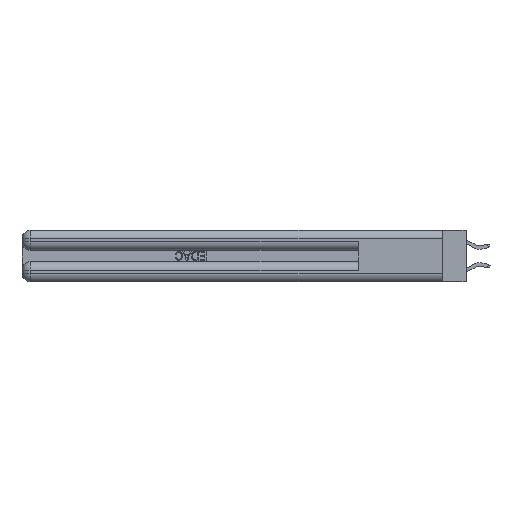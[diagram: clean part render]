
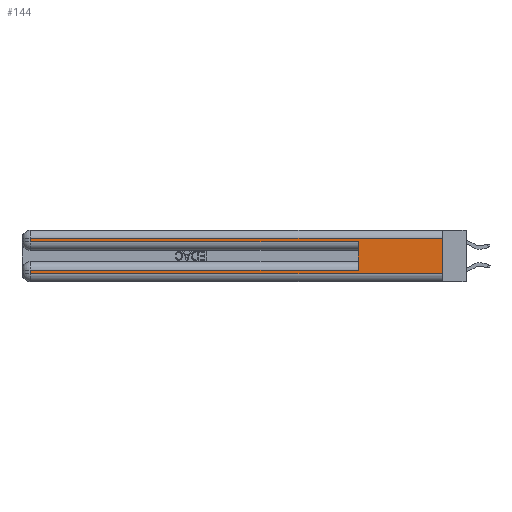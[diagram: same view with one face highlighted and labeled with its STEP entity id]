
A CAD part, left-side view. The second image highlights one B-rep face of the part: STEP entity #144.
In plain terms, the highlighted planar face has unit normal (-1, 0, 0).
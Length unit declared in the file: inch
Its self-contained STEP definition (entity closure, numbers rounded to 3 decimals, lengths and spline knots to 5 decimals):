
#144 = ADVANCED_FACE ( 'NONE', ( #13946 ), #8469, .F. ) ;
#1188 = CARTESIAN_POINT ( 'NONE',  ( 0., 2.94, 0.06 ) ) ;
#1198 = LINE ( 'NONE', #2480, #16249 ) ;
#1263 = ORIENTED_EDGE ( 'NONE', *, *, #7649, .T. ) ;
#2480 = CARTESIAN_POINT ( 'NONE',  ( 0., 2.94, 0.37 ) ) ;
#2558 = EDGE_CURVE ( 'NONE', #8866, #10875, #1198, .T. ) ;
#3335 = LINE ( 'NONE', #5764, #18402 ) ;
#3644 = VECTOR ( 'NONE', #9379, 39.37008 ) ;
#4234 = CARTESIAN_POINT ( 'NONE',  ( 0., 0., 0.31 ) ) ;
#4932 = CARTESIAN_POINT ( 'NONE',  ( 0., 0., 0.06 ) ) ;
#5012 = ORIENTED_EDGE ( 'NONE', *, *, #16796, .T. ) ;
#5206 = DIRECTION ( 'NONE',  ( 0., 0., -1. ) ) ;
#5764 = CARTESIAN_POINT ( 'NONE',  ( 0., 0., 0.285 ) ) ;
#6148 = DIRECTION ( 'NONE',  ( 0., 1., 0. ) ) ;
#6195 = EDGE_CURVE ( 'NONE', #19517, #17943, #30176, .T. ) ;
#6506 = EDGE_LOOP ( 'NONE', ( #23868, #1263, #18124, #16459, #20178, #26653, #28312, #5012 ) ) ;
#7344 = CARTESIAN_POINT ( 'NONE',  ( 0., 2.94, 0.085 ) ) ;
#7649 = EDGE_CURVE ( 'NONE', #25387, #8866, #16638, .T. ) ;
#8469 = PLANE ( 'NONE',  #24735 ) ;
#8866 = VERTEX_POINT ( 'NONE', #22800 ) ;
#9014 = CARTESIAN_POINT ( 'NONE',  ( 0., 0., 0.085 ) ) ;
#9054 = VECTOR ( 'NONE', #5206, 39.37008 ) ;
#9379 = DIRECTION ( 'NONE',  ( 0., -1., 0. ) ) ;
#9882 = VERTEX_POINT ( 'NONE', #25846 ) ;
#10875 = VERTEX_POINT ( 'NONE', #15319 ) ;
#11268 = EDGE_CURVE ( 'NONE', #10875, #9882, #3335, .T. ) ;
#12398 = DIRECTION ( 'NONE',  ( 0., 0., -1. ) ) ;
#13946 = FACE_OUTER_BOUND ( 'NONE', #6506, .T. ) ;
#14054 = CARTESIAN_POINT ( 'NONE',  ( 0., 0., 0.06 ) ) ;
#15319 = CARTESIAN_POINT ( 'NONE',  ( 0., 2.94, 0.285 ) ) ;
#16249 = VECTOR ( 'NONE', #26970, 39.37008 ) ;
#16356 = CARTESIAN_POINT ( 'NONE',  ( 0., 0., 0.37 ) ) ;
#16459 = ORIENTED_EDGE ( 'NONE', *, *, #11268, .T. ) ;
#16638 = LINE ( 'NONE', #4234, #23549 ) ;
#16796 = EDGE_CURVE ( 'NONE', #17943, #22755, #19067, .T. ) ;
#17441 = CARTESIAN_POINT ( 'NONE',  ( 0., 2.94, 0.37 ) ) ;
#17527 = CARTESIAN_POINT ( 'NONE',  ( 0., 0.6, 0.085 ) ) ;
#17943 = VERTEX_POINT ( 'NONE', #1188 ) ;
#18124 = ORIENTED_EDGE ( 'NONE', *, *, #2558, .T. ) ;
#18402 = VECTOR ( 'NONE', #20113, 39.37008 ) ;
#18943 = EDGE_CURVE ( 'NONE', #20857, #19517, #31115, .T. ) ;
#19067 = LINE ( 'NONE', #14054, #3644 ) ;
#19335 = VECTOR ( 'NONE', #12398, 39.37008 ) ;
#19431 = EDGE_CURVE ( 'NONE', #20857, #9882, #24582, .T. ) ;
#19517 = VERTEX_POINT ( 'NONE', #7344 ) ;
#19739 = CARTESIAN_POINT ( 'NONE',  ( 0., 0.6, 0.145 ) ) ;
#20113 = DIRECTION ( 'NONE',  ( 0., -1., 0. ) ) ;
#20178 = ORIENTED_EDGE ( 'NONE', *, *, #19431, .F. ) ;
#20857 = VERTEX_POINT ( 'NONE', #17527 ) ;
#22755 = VERTEX_POINT ( 'NONE', #4932 ) ;
#22800 = CARTESIAN_POINT ( 'NONE',  ( 0., 2.94, 0.31 ) ) ;
#23148 = DIRECTION ( 'NONE',  ( 1., 0., 0. ) ) ;
#23549 = VECTOR ( 'NONE', #31166, 39.37008 ) ;
#23868 = ORIENTED_EDGE ( 'NONE', *, *, #29521, .F. ) ;
#24582 = LINE ( 'NONE', #19739, #29580 ) ;
#24735 = AXIS2_PLACEMENT_3D ( 'NONE', #16356, #23148, #25875 ) ;
#25387 = VERTEX_POINT ( 'NONE', #28781 ) ;
#25846 = CARTESIAN_POINT ( 'NONE',  ( 0., 0.6, 0.285 ) ) ;
#25875 = DIRECTION ( 'NONE',  ( 0., 0., -1. ) ) ;
#26231 = DIRECTION ( 'NONE',  ( 0., 0., 1. ) ) ;
#26653 = ORIENTED_EDGE ( 'NONE', *, *, #18943, .T. ) ;
#26970 = DIRECTION ( 'NONE',  ( 0., 0., -1. ) ) ;
#28312 = ORIENTED_EDGE ( 'NONE', *, *, #6195, .T. ) ;
#28781 = CARTESIAN_POINT ( 'NONE',  ( 0., 0., 0.31 ) ) ;
#29343 = LINE ( 'NONE', #29482, #19335 ) ;
#29482 = CARTESIAN_POINT ( 'NONE',  ( 0., 0., 0.37 ) ) ;
#29521 = EDGE_CURVE ( 'NONE', #25387, #22755, #29343, .T. ) ;
#29580 = VECTOR ( 'NONE', #26231, 39.37008 ) ;
#30176 = LINE ( 'NONE', #17441, #9054 ) ;
#31095 = VECTOR ( 'NONE', #6148, 39.37008 ) ;
#31115 = LINE ( 'NONE', #9014, #31095 ) ;
#31166 = DIRECTION ( 'NONE',  ( 0., 1., 0. ) ) ;
